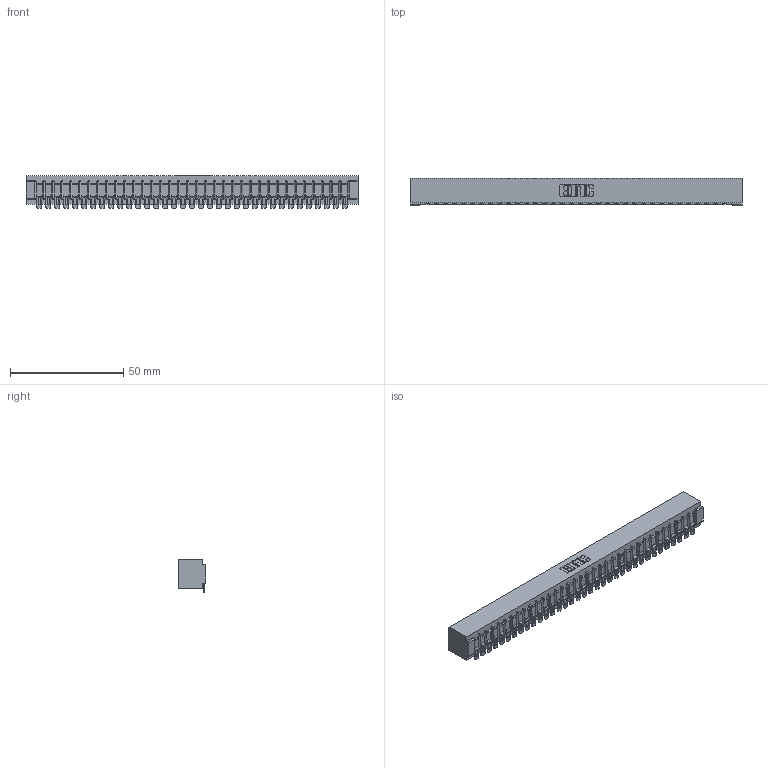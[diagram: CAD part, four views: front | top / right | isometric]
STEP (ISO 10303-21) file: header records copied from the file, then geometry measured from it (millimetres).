
FILE_DESCRIPTION (( 'STEP AP203' ), '1' );
FILE_NAME ('357-035-554-101.STEP', '2019-09-17T06:09:14', ( '' ), ( '' ), 'SwSTEP 2.0', 'SolidWorks 2016', '' );
FILE_SCHEMA (( 'CONFIG_CONTROL_DESIGN' ));
Length unit declared in the file: inch
Products named in the file (3): 307-290-002_554; 357-035-554-101; 307 Part_No Mounting Lugs
Assembly tree (36 placements, depth 2):
  357-035-554-101
    307 Part_No Mounting Lugs
    307-290-002_554  x35
Bounding box: 146.56 x 12.01 x 14.52 mm (x, y, z)
Volume: 16201.7 mm3; surface area: 20702.5 mm2
Topology: 36 solids, 36 shells, 2981 faces, 9154 edges, 6004 vertices
Faces by surface type: plane 1676, cylinder 1233, sphere 72
Entity records: 31555 total; most frequent: CARTESIAN_POINT 5322, ORIENTED_EDGE 5312, DIRECTION 5178, EDGE_CURVE 2656, LINE 2026, VECTOR 2026, VERTEX_POINT 1720, AXIS2_PLACEMENT_3D 1576
